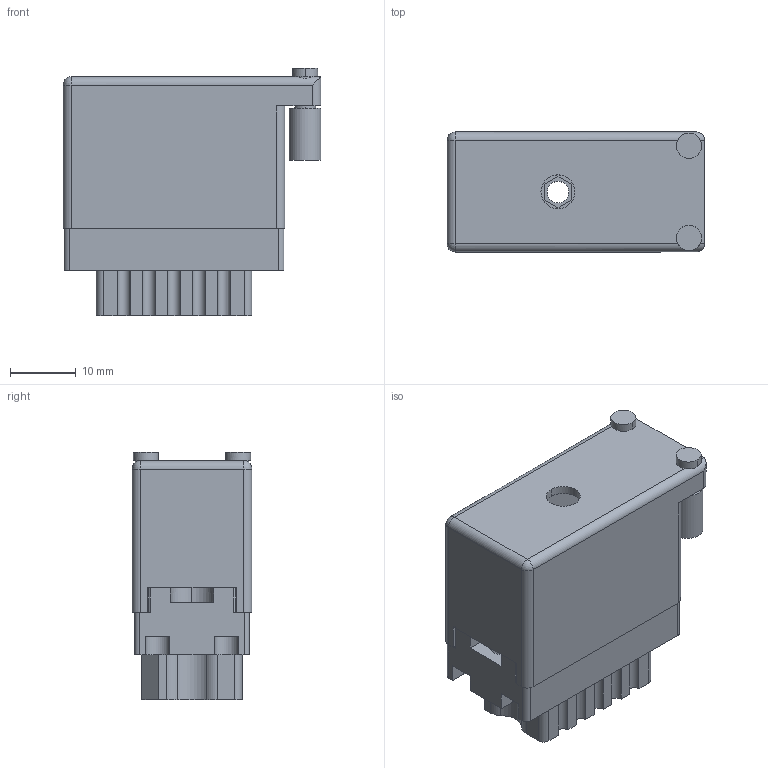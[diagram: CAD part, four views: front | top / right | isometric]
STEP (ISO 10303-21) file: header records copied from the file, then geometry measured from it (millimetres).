
FILE_DESCRIPTION (( 'STEP AP203' ), '1' );
FILE_NAME ('519-014-501-450.STEP', '2020-09-09T18:32:55', ( '' ), ( '' ), 'SwSTEP 2.0', 'SolidWorks 2020', '' );
FILE_SCHEMA (( 'CONFIG_CONTROL_DESIGN' ));
Length unit declared in the file: inch
Products named in the file (4): 516-230-001_Metal - 020 Side Entry; 519 Receptacle Insulator_014; 516-292-001_501 Contact; 519-014-501-450
Assembly tree (16 placements, depth 2):
  519-014-501-450
    519 Receptacle Insulator_014
    516-292-001_501 Contact  x14
    516-230-001_Metal - 020 Side Entry
Bounding box: 39.12 x 18.16 x 37.52 mm (x, y, z)
Volume: 10470.7 mm3; surface area: 15311.2 mm2
Topology: 16 solids, 16 shells, 1551 faces, 4484 edges, 2972 vertices
Faces by surface type: plane 932, cylinder 531, bspline 84, cone 2, sphere 2
Entity records: 21375 total; most frequent: CARTESIAN_POINT 3912, ORIENTED_EDGE 3556, DIRECTION 3460, EDGE_CURVE 1778, VECTOR 1274, LINE 1274, VERTEX_POINT 1178, AXIS2_PLACEMENT_3D 1093
